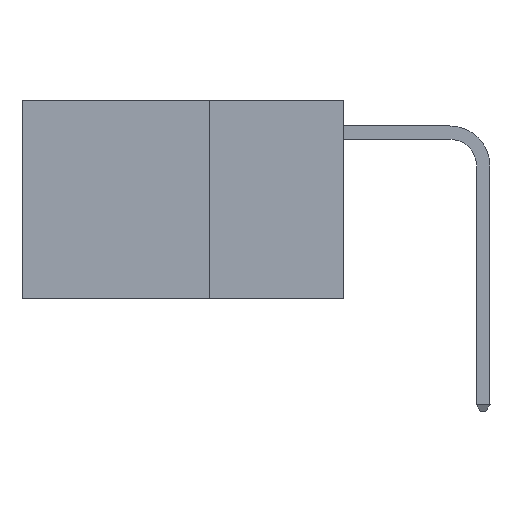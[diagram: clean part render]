
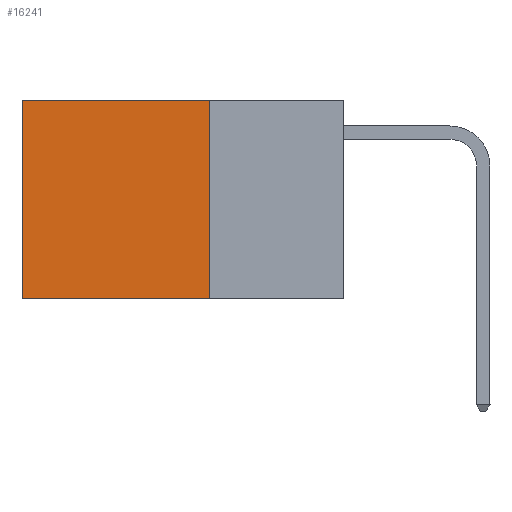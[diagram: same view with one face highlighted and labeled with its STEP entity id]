
A CAD part, left-side view. The second image highlights one B-rep face of the part: STEP entity #16241.
In plain terms, the highlighted planar face has unit normal (-1, 0, 0).
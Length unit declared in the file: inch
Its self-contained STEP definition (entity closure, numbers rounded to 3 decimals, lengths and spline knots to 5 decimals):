
#470 = CARTESIAN_POINT ( 'NONE',  ( 0.2625, 0.25, 0. ) ) ;
#1490 = DIRECTION ( 'NONE',  ( 0., 1., 0. ) ) ;
#2243 = ORIENTED_EDGE ( 'NONE', *, *, #13744, .T. ) ;
#2952 = EDGE_CURVE ( 'NONE', #17666, #3960, #27455, .T. ) ;
#3220 = VERTEX_POINT ( 'NONE', #470 ) ;
#3379 = FACE_OUTER_BOUND ( 'NONE', #14080, .T. ) ;
#3546 = DIRECTION ( 'NONE',  ( 0., 0., -1. ) ) ;
#3960 = VERTEX_POINT ( 'NONE', #23131 ) ;
#4061 = VECTOR ( 'NONE', #13833, 39.37008 ) ;
#5128 = CARTESIAN_POINT ( 'NONE',  ( 0.2625, 0.25, 0. ) ) ;
#5404 = LINE ( 'NONE', #5128, #4061 ) ;
#5501 = VECTOR ( 'NONE', #1490, 39.37008 ) ;
#6469 = AXIS2_PLACEMENT_3D ( 'NONE', #13926, #21014, #27115 ) ;
#6576 = DIRECTION ( 'NONE',  ( 0., 1., 0. ) ) ;
#10061 = PLANE ( 'NONE',  #6469 ) ;
#10367 = CARTESIAN_POINT ( 'NONE',  ( 0.2625, 0.6, 0. ) ) ;
#11088 = EDGE_CURVE ( 'NONE', #3220, #17666, #5404, .T. ) ;
#11587 = VECTOR ( 'NONE', #3546, 39.37008 ) ;
#13261 = VECTOR ( 'NONE', #6576, 39.37008 ) ;
#13744 = EDGE_CURVE ( 'NONE', #3220, #14659, #17394, .T. ) ;
#13833 = DIRECTION ( 'NONE',  ( 0., 0., -1. ) ) ;
#13926 = CARTESIAN_POINT ( 'NONE',  ( 0.2625, 0.25, 0. ) ) ;
#14080 = EDGE_LOOP ( 'NONE', ( #17455, #26286, #25277, #2243 ) ) ;
#14659 = VERTEX_POINT ( 'NONE', #10367 ) ;
#16241 = ADVANCED_FACE ( 'NONE', ( #3379 ), #10061, .F. ) ;
#16380 = CARTESIAN_POINT ( 'NONE',  ( 0.2625, 0.25, -0.37 ) ) ;
#17394 = LINE ( 'NONE', #21655, #13261 ) ;
#17455 = ORIENTED_EDGE ( 'NONE', *, *, #21359, .T. ) ;
#17666 = VERTEX_POINT ( 'NONE', #26283 ) ;
#18895 = LINE ( 'NONE', #27556, #11587 ) ;
#21014 = DIRECTION ( 'NONE',  ( 1., 0., 0. ) ) ;
#21359 = EDGE_CURVE ( 'NONE', #14659, #3960, #18895, .T. ) ;
#21655 = CARTESIAN_POINT ( 'NONE',  ( 0.2625, 0.25, 0. ) ) ;
#23131 = CARTESIAN_POINT ( 'NONE',  ( 0.2625, 0.6, -0.37 ) ) ;
#25277 = ORIENTED_EDGE ( 'NONE', *, *, #11088, .F. ) ;
#26283 = CARTESIAN_POINT ( 'NONE',  ( 0.2625, 0.25, -0.37 ) ) ;
#26286 = ORIENTED_EDGE ( 'NONE', *, *, #2952, .F. ) ;
#27115 = DIRECTION ( 'NONE',  ( 0., 0., -1. ) ) ;
#27455 = LINE ( 'NONE', #16380, #5501 ) ;
#27556 = CARTESIAN_POINT ( 'NONE',  ( 0.2625, 0.6, 0. ) ) ;
